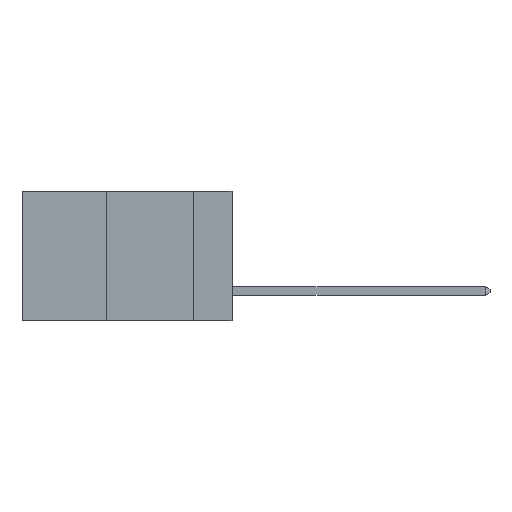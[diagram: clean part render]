
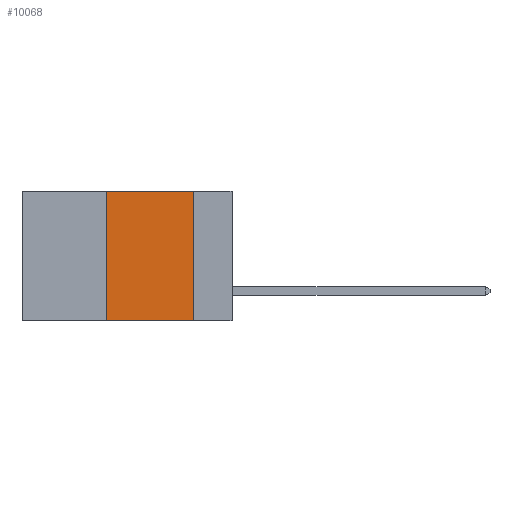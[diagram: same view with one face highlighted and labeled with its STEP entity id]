
A CAD part, left-side view. The second image highlights one B-rep face of the part: STEP entity #10068.
In plain terms, the highlighted planar face has unit normal (-1, 0, 0).
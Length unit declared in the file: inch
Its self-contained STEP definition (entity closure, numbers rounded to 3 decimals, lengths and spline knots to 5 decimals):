
#399 = AXIS2_PLACEMENT_3D ( 'NONE', #1819, #9787, #3065 ) ;
#1201 = EDGE_LOOP ( 'NONE', ( #6556, #4181, #7243, #1308 ) ) ;
#1308 = ORIENTED_EDGE ( 'NONE', *, *, #14021, .T. ) ;
#1819 = CARTESIAN_POINT ( 'NONE',  ( 0., 0.6, 0. ) ) ;
#2483 = VERTEX_POINT ( 'NONE', #7868 ) ;
#2496 = CARTESIAN_POINT ( 'NONE',  ( 0., 0.36, 0. ) ) ;
#3057 = CARTESIAN_POINT ( 'NONE',  ( 0., 0.6, 0. ) ) ;
#3065 = DIRECTION ( 'NONE',  ( 0., 0., -1. ) ) ;
#3211 = LINE ( 'NONE', #7705, #8213 ) ;
#3220 = CARTESIAN_POINT ( 'NONE',  ( 0., 0.36, 0. ) ) ;
#3290 = FACE_OUTER_BOUND ( 'NONE', #1201, .T. ) ;
#4181 = ORIENTED_EDGE ( 'NONE', *, *, #4346, .F. ) ;
#4346 = EDGE_CURVE ( 'NONE', #13031, #4435, #5426, .T. ) ;
#4435 = VERTEX_POINT ( 'NONE', #12775 ) ;
#4673 = VECTOR ( 'NONE', #10971, 39.37008 ) ;
#5369 = VERTEX_POINT ( 'NONE', #6778 ) ;
#5426 = LINE ( 'NONE', #3057, #4673 ) ;
#6081 = LINE ( 'NONE', #10576, #11414 ) ;
#6556 = ORIENTED_EDGE ( 'NONE', *, *, #10430, .F. ) ;
#6778 = CARTESIAN_POINT ( 'NONE',  ( 0., 0.11, -0.37 ) ) ;
#7243 = ORIENTED_EDGE ( 'NONE', *, *, #14096, .F. ) ;
#7705 = CARTESIAN_POINT ( 'NONE',  ( 0., 0.6, -0.37 ) ) ;
#7868 = CARTESIAN_POINT ( 'NONE',  ( 0., 0.36, -0.37 ) ) ;
#7875 = LINE ( 'NONE', #3220, #10369 ) ;
#8213 = VECTOR ( 'NONE', #8796, 39.37008 ) ;
#8751 = PLANE ( 'NONE',  #399 ) ;
#8796 = DIRECTION ( 'NONE',  ( 0., -1., 0. ) ) ;
#9787 = DIRECTION ( 'NONE',  ( 1., 0., 0. ) ) ;
#10068 = ADVANCED_FACE ( 'NONE', ( #3290 ), #8751, .F. ) ;
#10369 = VECTOR ( 'NONE', #12002, 39.37008 ) ;
#10430 = EDGE_CURVE ( 'NONE', #4435, #5369, #6081, .T. ) ;
#10576 = CARTESIAN_POINT ( 'NONE',  ( 0., 0.11, 0. ) ) ;
#10971 = DIRECTION ( 'NONE',  ( 0., -1., 0. ) ) ;
#11414 = VECTOR ( 'NONE', #11600, 39.37008 ) ;
#11600 = DIRECTION ( 'NONE',  ( 0., 0., -1. ) ) ;
#12002 = DIRECTION ( 'NONE',  ( 0., 0., 1. ) ) ;
#12775 = CARTESIAN_POINT ( 'NONE',  ( 0., 0.11, 0. ) ) ;
#13031 = VERTEX_POINT ( 'NONE', #2496 ) ;
#14021 = EDGE_CURVE ( 'NONE', #2483, #5369, #3211, .T. ) ;
#14096 = EDGE_CURVE ( 'NONE', #2483, #13031, #7875, .T. ) ;
